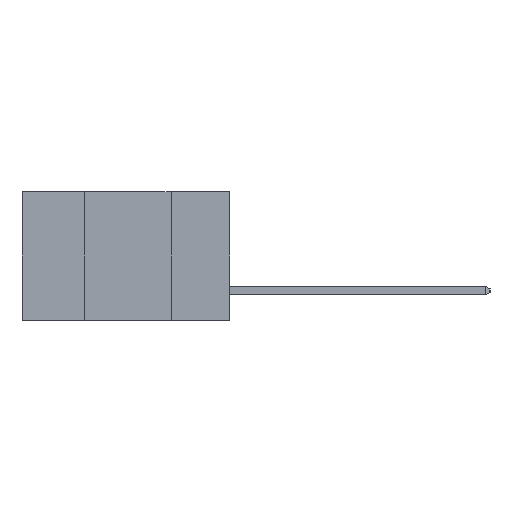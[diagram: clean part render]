
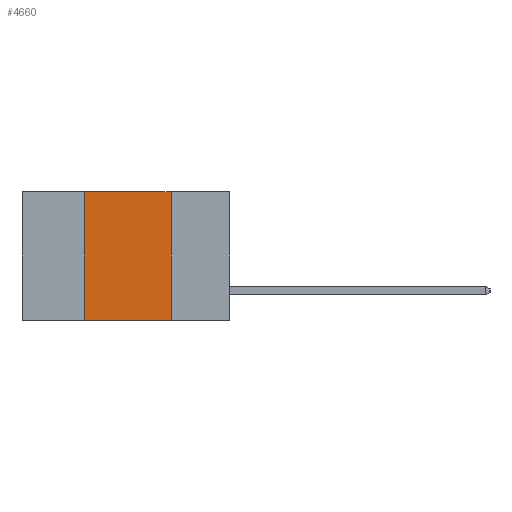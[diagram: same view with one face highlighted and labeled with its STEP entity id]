
A CAD part, left-side view. The second image highlights one B-rep face of the part: STEP entity #4660.
In plain terms, the highlighted planar face has unit normal (-1, 0, 0).
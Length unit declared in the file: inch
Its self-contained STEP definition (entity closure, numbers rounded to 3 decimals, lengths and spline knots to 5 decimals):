
#790 = LINE ( 'NONE', #15030, #13205 ) ;
#1086 = DIRECTION ( 'NONE',  ( 0., -1., 0. ) ) ;
#1361 = ORIENTED_EDGE ( 'NONE', *, *, #4044, .F. ) ;
#2119 = ORIENTED_EDGE ( 'NONE', *, *, #4062, .T. ) ;
#3573 = VERTEX_POINT ( 'NONE', #14691 ) ;
#3729 = VERTEX_POINT ( 'NONE', #6413 ) ;
#4011 = ORIENTED_EDGE ( 'NONE', *, *, #4042, .F. ) ;
#4042 = EDGE_CURVE ( 'NONE', #8339, #3573, #790, .T. ) ;
#4044 = EDGE_CURVE ( 'NONE', #3729, #11009, #4183, .T. ) ;
#4062 = EDGE_CURVE ( 'NONE', #3729, #3573, #9849, .T. ) ;
#4178 = AXIS2_PLACEMENT_3D ( 'NONE', #8185, #5839, #5646 ) ;
#4183 = LINE ( 'NONE', #14416, #10588 ) ;
#4307 = EDGE_LOOP ( 'NONE', ( #4011, #4554, #1361, #2119 ) ) ;
#4410 = LINE ( 'NONE', #6147, #7335 ) ;
#4554 = ORIENTED_EDGE ( 'NONE', *, *, #12891, .F. ) ;
#4660 = ADVANCED_FACE ( 'NONE', ( #8537 ), #13425, .F. ) ;
#5646 = DIRECTION ( 'NONE',  ( 0., 0., -1. ) ) ;
#5839 = DIRECTION ( 'NONE',  ( 1., 0., 0. ) ) ;
#6147 = CARTESIAN_POINT ( 'NONE',  ( 0., 0.6, 0. ) ) ;
#6413 = CARTESIAN_POINT ( 'NONE',  ( 0., 0.42, -0.37 ) ) ;
#7131 = VECTOR ( 'NONE', #11596, 39.37008 ) ;
#7335 = VECTOR ( 'NONE', #1086, 39.37008 ) ;
#8185 = CARTESIAN_POINT ( 'NONE',  ( 0., 0.6, 0. ) ) ;
#8339 = VERTEX_POINT ( 'NONE', #8600 ) ;
#8537 = FACE_OUTER_BOUND ( 'NONE', #4307, .T. ) ;
#8600 = CARTESIAN_POINT ( 'NONE',  ( 0., 0.17, 0. ) ) ;
#9849 = LINE ( 'NONE', #11615, #7131 ) ;
#10588 = VECTOR ( 'NONE', #10725, 39.37008 ) ;
#10725 = DIRECTION ( 'NONE',  ( 0., 0., 1. ) ) ;
#10927 = CARTESIAN_POINT ( 'NONE',  ( 0., 0.42, 0. ) ) ;
#11009 = VERTEX_POINT ( 'NONE', #10927 ) ;
#11596 = DIRECTION ( 'NONE',  ( 0., -1., 0. ) ) ;
#11615 = CARTESIAN_POINT ( 'NONE',  ( 0., 0.6, -0.37 ) ) ;
#12891 = EDGE_CURVE ( 'NONE', #11009, #8339, #4410, .T. ) ;
#13205 = VECTOR ( 'NONE', #14875, 39.37008 ) ;
#13425 = PLANE ( 'NONE',  #4178 ) ;
#14416 = CARTESIAN_POINT ( 'NONE',  ( 0., 0.42, 0. ) ) ;
#14691 = CARTESIAN_POINT ( 'NONE',  ( 0., 0.17, -0.37 ) ) ;
#14875 = DIRECTION ( 'NONE',  ( 0., 0., -1. ) ) ;
#15030 = CARTESIAN_POINT ( 'NONE',  ( 0., 0.17, 0. ) ) ;
